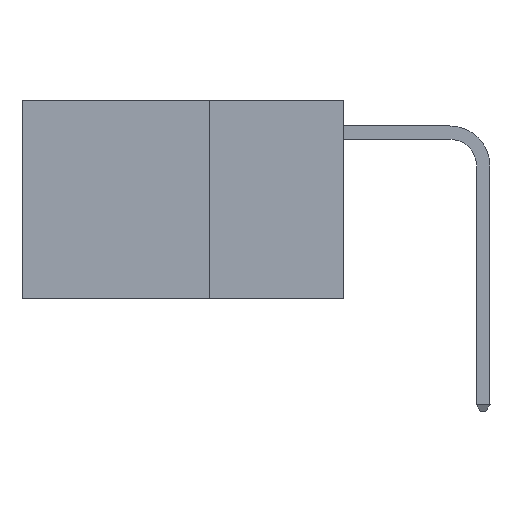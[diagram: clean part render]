
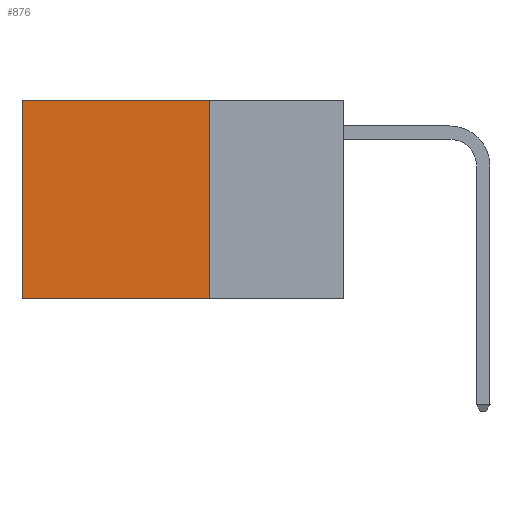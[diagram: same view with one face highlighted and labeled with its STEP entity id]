
A CAD part, left-side view. The second image highlights one B-rep face of the part: STEP entity #876.
In plain terms, the highlighted planar face has unit normal (-1, 0, 0).
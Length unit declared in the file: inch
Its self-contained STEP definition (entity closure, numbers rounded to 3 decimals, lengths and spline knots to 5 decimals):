
#332 = DIRECTION ( 'NONE',  ( 1., 0., 0. ) ) ;
#345 = ORIENTED_EDGE ( 'NONE', *, *, #729, .T. ) ;
#729 = EDGE_CURVE ( 'NONE', #4180, #8387, #11196, .T. ) ;
#864 = PLANE ( 'NONE',  #14628 ) ;
#876 = ADVANCED_FACE ( 'NONE', ( #9934 ), #864, .F. ) ;
#1378 = VERTEX_POINT ( 'NONE', #14086 ) ;
#1776 = CARTESIAN_POINT ( 'NONE',  ( 0.2625, 0.6, 0. ) ) ;
#1899 = LINE ( 'NONE', #4456, #16271 ) ;
#1912 = DIRECTION ( 'NONE',  ( 0., 0., -1. ) ) ;
#1933 = CARTESIAN_POINT ( 'NONE',  ( 0.2625, 0.25, 0. ) ) ;
#2230 = CARTESIAN_POINT ( 'NONE',  ( 0.2625, 0.6, -0.37 ) ) ;
#2312 = VECTOR ( 'NONE', #5592, 39.37008 ) ;
#4143 = VECTOR ( 'NONE', #1912, 39.37008 ) ;
#4180 = VERTEX_POINT ( 'NONE', #1776 ) ;
#4187 = LINE ( 'NONE', #1933, #4143 ) ;
#4252 = DIRECTION ( 'NONE',  ( 0., 1., 0. ) ) ;
#4313 = CARTESIAN_POINT ( 'NONE',  ( 0.2625, 0.25, 0. ) ) ;
#4456 = CARTESIAN_POINT ( 'NONE',  ( 0.2625, 0.25, 0. ) ) ;
#4886 = DIRECTION ( 'NONE',  ( 0., 0., -1. ) ) ;
#5140 = DIRECTION ( 'NONE',  ( 0., 0., -1. ) ) ;
#5592 = DIRECTION ( 'NONE',  ( 0., 1., 0. ) ) ;
#6599 = ORIENTED_EDGE ( 'NONE', *, *, #8154, .T. ) ;
#8154 = EDGE_CURVE ( 'NONE', #1378, #4180, #1899, .T. ) ;
#8387 = VERTEX_POINT ( 'NONE', #2230 ) ;
#8431 = ORIENTED_EDGE ( 'NONE', *, *, #15831, .F. ) ;
#8476 = EDGE_LOOP ( 'NONE', ( #345, #8431, #8722, #6599 ) ) ;
#8722 = ORIENTED_EDGE ( 'NONE', *, *, #10605, .F. ) ;
#9676 = LINE ( 'NONE', #11974, #2312 ) ;
#9934 = FACE_OUTER_BOUND ( 'NONE', #8476, .T. ) ;
#10398 = CARTESIAN_POINT ( 'NONE',  ( 0.2625, 0.6, 0. ) ) ;
#10605 = EDGE_CURVE ( 'NONE', #1378, #12843, #4187, .T. ) ;
#11110 = VECTOR ( 'NONE', #5140, 39.37008 ) ;
#11196 = LINE ( 'NONE', #10398, #11110 ) ;
#11974 = CARTESIAN_POINT ( 'NONE',  ( 0.2625, 0.25, -0.37 ) ) ;
#12843 = VERTEX_POINT ( 'NONE', #14602 ) ;
#14086 = CARTESIAN_POINT ( 'NONE',  ( 0.2625, 0.25, 0. ) ) ;
#14602 = CARTESIAN_POINT ( 'NONE',  ( 0.2625, 0.25, -0.37 ) ) ;
#14628 = AXIS2_PLACEMENT_3D ( 'NONE', #4313, #332, #4886 ) ;
#15831 = EDGE_CURVE ( 'NONE', #12843, #8387, #9676, .T. ) ;
#16271 = VECTOR ( 'NONE', #4252, 39.37008 ) ;
